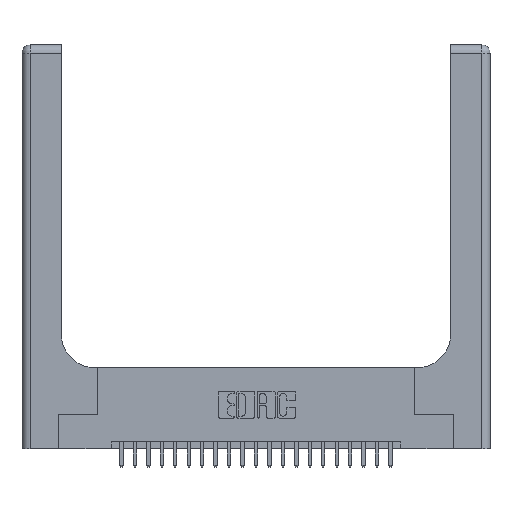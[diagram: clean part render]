
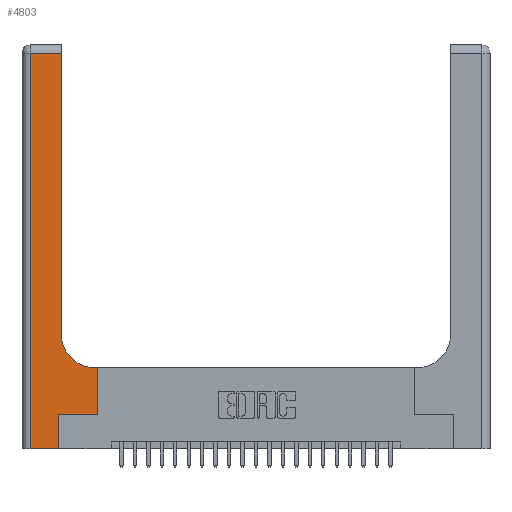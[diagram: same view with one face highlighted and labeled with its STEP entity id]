
A CAD part, top view. The second image highlights one B-rep face of the part: STEP entity #4803.
In plain terms, the highlighted planar face has unit normal (0, 0, 1).
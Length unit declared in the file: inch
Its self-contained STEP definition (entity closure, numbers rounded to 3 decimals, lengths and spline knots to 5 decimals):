
#1428 = DIRECTION ( 'NONE',  ( 0., 1., 0. ) ) ;
#2036 = CARTESIAN_POINT ( 'NONE',  ( 0., 3., 0.37 ) ) ;
#2479 = ORIENTED_EDGE ( 'NONE', *, *, #15204, .T. ) ;
#2649 = EDGE_CURVE ( 'NONE', #20390, #19859, #5396, .T. ) ;
#3019 = VERTEX_POINT ( 'NONE', #10227 ) ;
#3078 = CIRCLE ( 'NONE', #24106, 0.25 ) ;
#3380 = EDGE_CURVE ( 'NONE', #19859, #20222, #5055, .T. ) ;
#3731 = CARTESIAN_POINT ( 'NONE',  ( 0.269, 0., 0.37 ) ) ;
#3871 = CARTESIAN_POINT ( 'NONE',  ( 0.5585, 0.6, 0.37 ) ) ;
#3985 = DIRECTION ( 'NONE',  ( 0., 0., -1. ) ) ;
#4078 = ORIENTED_EDGE ( 'NONE', *, *, #3380, .T. ) ;
#4744 = VERTEX_POINT ( 'NONE', #13402 ) ;
#4792 = DIRECTION ( 'NONE',  ( 1., 0., 0. ) ) ;
#4803 = ADVANCED_FACE ( 'NONE', ( #22580 ), #13493, .F. ) ;
#5055 = LINE ( 'NONE', #11140, #19600 ) ;
#5126 = VECTOR ( 'NONE', #17782, 39.37008 ) ;
#5383 = VERTEX_POINT ( 'NONE', #15692 ) ;
#5396 = LINE ( 'NONE', #18331, #11130 ) ;
#7064 = VERTEX_POINT ( 'NONE', #3871 ) ;
#7676 = CARTESIAN_POINT ( 'NONE',  ( 0.5415, 0.6, 0.37 ) ) ;
#8450 = VECTOR ( 'NONE', #18372, 39.37008 ) ;
#8531 = EDGE_CURVE ( 'NONE', #5383, #11032, #14941, .T. ) ;
#9400 = DIRECTION ( 'NONE',  ( -1., 0., 0. ) ) ;
#9658 = LINE ( 'NONE', #10892, #8450 ) ;
#9820 = DIRECTION ( 'NONE',  ( 0., 0., -1. ) ) ;
#9957 = CARTESIAN_POINT ( 'NONE',  ( 0.2915, 0.6, 0.37 ) ) ;
#10227 = CARTESIAN_POINT ( 'NONE',  ( 0.2915, 0.85, 0.37 ) ) ;
#10618 = EDGE_LOOP ( 'NONE', ( #2479, #11250, #13006, #19145, #4078, #14016, #12835, #22952, #17787 ) ) ;
#10688 = VECTOR ( 'NONE', #13805, 39.37008 ) ;
#10759 = DIRECTION ( 'NONE',  ( 1., 0., 0. ) ) ;
#10783 = EDGE_CURVE ( 'NONE', #11032, #20390, #9658, .T. ) ;
#10852 = LINE ( 'NONE', #15933, #5126 ) ;
#10892 = CARTESIAN_POINT ( 'NONE',  ( 0.06, 3., 0.37 ) ) ;
#11032 = VERTEX_POINT ( 'NONE', #24296 ) ;
#11066 = VECTOR ( 'NONE', #9400, 39.37008 ) ;
#11130 = VECTOR ( 'NONE', #10759, 39.37008 ) ;
#11140 = CARTESIAN_POINT ( 'NONE',  ( 0.269, 0., 0.37 ) ) ;
#11250 = ORIENTED_EDGE ( 'NONE', *, *, #8531, .T. ) ;
#11283 = LINE ( 'NONE', #9957, #10688 ) ;
#12409 = DIRECTION ( 'NONE',  ( 0., 1., 0. ) ) ;
#12835 = ORIENTED_EDGE ( 'NONE', *, *, #17461, .T. ) ;
#13006 = ORIENTED_EDGE ( 'NONE', *, *, #10783, .T. ) ;
#13402 = CARTESIAN_POINT ( 'NONE',  ( 0.5585, 0.25, 0.37 ) ) ;
#13493 = PLANE ( 'NONE',  #19554 ) ;
#13805 = DIRECTION ( 'NONE',  ( -1., 0., 0. ) ) ;
#14016 = ORIENTED_EDGE ( 'NONE', *, *, #16413, .T. ) ;
#14816 = LINE ( 'NONE', #18099, #19133 ) ;
#14941 = LINE ( 'NONE', #18798, #11066 ) ;
#14990 = CARTESIAN_POINT ( 'NONE',  ( 0.06, 0., 0.37 ) ) ;
#15204 = EDGE_CURVE ( 'NONE', #3019, #5383, #16328, .T. ) ;
#15692 = CARTESIAN_POINT ( 'NONE',  ( 0.2915, 2.94, 0.37 ) ) ;
#15738 = VECTOR ( 'NONE', #12409, 39.37008 ) ;
#15933 = CARTESIAN_POINT ( 'NONE',  ( 0.5585, 0.25, 0.37 ) ) ;
#16328 = LINE ( 'NONE', #19863, #15738 ) ;
#16413 = EDGE_CURVE ( 'NONE', #20222, #4744, #14816, .T. ) ;
#17334 = DIRECTION ( 'NONE',  ( -1., 0., 0. ) ) ;
#17461 = EDGE_CURVE ( 'NONE', #4744, #7064, #10852, .T. ) ;
#17782 = DIRECTION ( 'NONE',  ( 0., 1., 0. ) ) ;
#17787 = ORIENTED_EDGE ( 'NONE', *, *, #21719, .T. ) ;
#18099 = CARTESIAN_POINT ( 'NONE',  ( 0.269, 0.25, 0.37 ) ) ;
#18331 = CARTESIAN_POINT ( 'NONE',  ( 0., 0., 0.37 ) ) ;
#18372 = DIRECTION ( 'NONE',  ( 0., -1., 0. ) ) ;
#18798 = CARTESIAN_POINT ( 'NONE',  ( 0., 2.94, 0.37 ) ) ;
#19133 = VECTOR ( 'NONE', #4792, 39.37008 ) ;
#19145 = ORIENTED_EDGE ( 'NONE', *, *, #2649, .T. ) ;
#19554 = AXIS2_PLACEMENT_3D ( 'NONE', #2036, #3985, #17334 ) ;
#19600 = VECTOR ( 'NONE', #1428, 39.37008 ) ;
#19859 = VERTEX_POINT ( 'NONE', #3731 ) ;
#19863 = CARTESIAN_POINT ( 'NONE',  ( 0.2915, 3., 0.37 ) ) ;
#20222 = VERTEX_POINT ( 'NONE', #21839 ) ;
#20390 = VERTEX_POINT ( 'NONE', #14990 ) ;
#20556 = VERTEX_POINT ( 'NONE', #7676 ) ;
#20675 = EDGE_CURVE ( 'NONE', #7064, #20556, #11283, .T. ) ;
#21041 = CARTESIAN_POINT ( 'NONE',  ( 0.5415, 0.85, 0.37 ) ) ;
#21719 = EDGE_CURVE ( 'NONE', #20556, #3019, #3078, .T. ) ;
#21839 = CARTESIAN_POINT ( 'NONE',  ( 0.269, 0.25, 0.37 ) ) ;
#22580 = FACE_OUTER_BOUND ( 'NONE', #10618, .T. ) ;
#22883 = DIRECTION ( 'NONE',  ( 1., 0., 0. ) ) ;
#22952 = ORIENTED_EDGE ( 'NONE', *, *, #20675, .T. ) ;
#24106 = AXIS2_PLACEMENT_3D ( 'NONE', #21041, #9820, #22883 ) ;
#24296 = CARTESIAN_POINT ( 'NONE',  ( 0.06, 2.94, 0.37 ) ) ;
